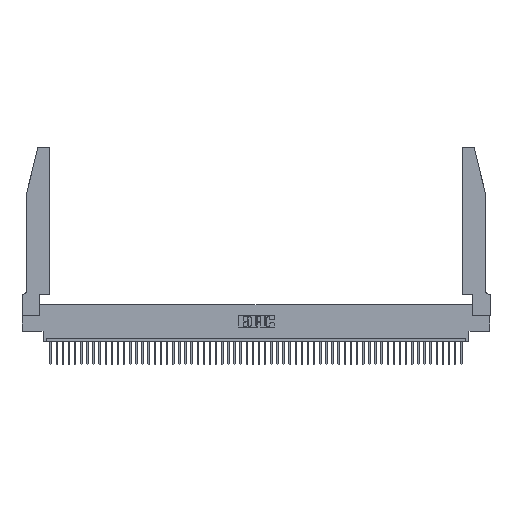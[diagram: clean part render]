
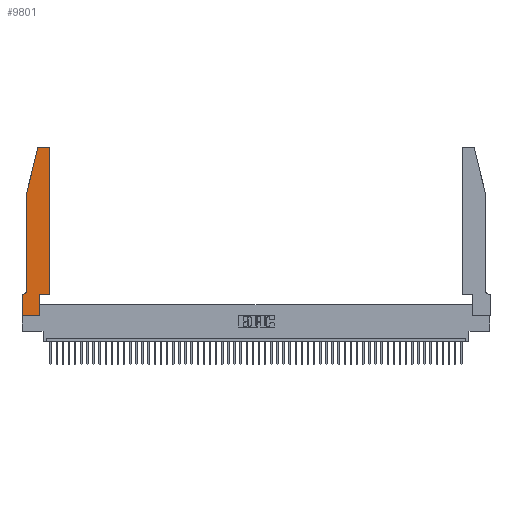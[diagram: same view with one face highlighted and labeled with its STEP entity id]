
A CAD part, top view. The second image highlights one B-rep face of the part: STEP entity #9801.
In plain terms, the highlighted planar face has unit normal (0, 0, 1).
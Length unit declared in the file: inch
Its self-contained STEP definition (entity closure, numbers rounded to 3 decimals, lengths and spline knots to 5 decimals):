
#990 = CARTESIAN_POINT ( 'NONE',  ( 0.2605, 2.75, 0.37 ) ) ;
#1008 = DIRECTION ( 'NONE',  ( 1., 0., 0. ) ) ;
#2313 = ORIENTED_EDGE ( 'NONE', *, *, #16803, .T. ) ;
#2645 = CARTESIAN_POINT ( 'NONE',  ( 0.0755, 0.42, 0.37 ) ) ;
#2916 = VECTOR ( 'NONE', #13796, 39.37008 ) ;
#2956 = DIRECTION ( 'NONE',  ( 0., 1., 0. ) ) ;
#4282 = VECTOR ( 'NONE', #18488, 39.37008 ) ;
#5084 = EDGE_CURVE ( 'NONE', #20012, #34031, #16557, .T. ) ;
#5178 = EDGE_CURVE ( 'NONE', #34031, #5713, #45083, .T. ) ;
#5594 = DIRECTION ( 'NONE',  ( 0., 0., 1. ) ) ;
#5713 = VERTEX_POINT ( 'NONE', #12394 ) ;
#6155 = EDGE_CURVE ( 'NONE', #8151, #35009, #12959, .T. ) ;
#7456 = VECTOR ( 'NONE', #34165, 39.37008 ) ;
#8151 = VERTEX_POINT ( 'NONE', #10518 ) ;
#9075 = CARTESIAN_POINT ( 'NONE',  ( 0.2865, 0.35, 0.37 ) ) ;
#9334 = CARTESIAN_POINT ( 'NONE',  ( 0., 0., 0.37 ) ) ;
#9801 = ADVANCED_FACE ( 'NONE', ( #12175 ), #47175, .T. ) ;
#10412 = ORIENTED_EDGE ( 'NONE', *, *, #41816, .T. ) ;
#10518 = CARTESIAN_POINT ( 'NONE',  ( 0.0755, 2., 0.37 ) ) ;
#11980 = CARTESIAN_POINT ( 'NONE',  ( 0.4205, 2.75, 0.37 ) ) ;
#12064 = CIRCLE ( 'NONE', #22218, 0.03 ) ;
#12175 = FACE_OUTER_BOUND ( 'NONE', #51676, .T. ) ;
#12394 = CARTESIAN_POINT ( 'NONE',  ( 0., 0., 0.37 ) ) ;
#12959 = LINE ( 'NONE', #13630, #49100 ) ;
#13179 = EDGE_CURVE ( 'NONE', #5713, #50501, #47459, .T. ) ;
#13371 = EDGE_CURVE ( 'NONE', #25497, #16295, #32127, .T. ) ;
#13630 = CARTESIAN_POINT ( 'NONE',  ( 0.0755, 2., 0.37 ) ) ;
#13796 = DIRECTION ( 'NONE',  ( 1., 0., 0. ) ) ;
#14965 = LINE ( 'NONE', #47362, #35889 ) ;
#16295 = VERTEX_POINT ( 'NONE', #37887 ) ;
#16557 = LINE ( 'NONE', #52510, #31771 ) ;
#16803 = EDGE_CURVE ( 'NONE', #27296, #44970, #12064, .T. ) ;
#17309 = VECTOR ( 'NONE', #37093, 39.37008 ) ;
#17641 = CARTESIAN_POINT ( 'NONE',  ( 0.4205, 2.72, 0.37 ) ) ;
#18488 = DIRECTION ( 'NONE',  ( -0.239, -0.971, 0. ) ) ;
#18759 = CARTESIAN_POINT ( 'NONE',  ( 0.2865, 0., 0.37 ) ) ;
#19141 = CARTESIAN_POINT ( 'NONE',  ( 0., 0.35, 0.37 ) ) ;
#20012 = VERTEX_POINT ( 'NONE', #29190 ) ;
#20167 = DIRECTION ( 'NONE',  ( -1., 0., 0. ) ) ;
#20711 = LINE ( 'NONE', #990, #7456 ) ;
#21055 = CIRCLE ( 'NONE', #21186, 0.03 ) ;
#21186 = AXIS2_PLACEMENT_3D ( 'NONE', #29906, #5594, #1008 ) ;
#21304 = ORIENTED_EDGE ( 'NONE', *, *, #41875, .T. ) ;
#21490 = DIRECTION ( 'NONE',  ( 1., 0., 0. ) ) ;
#22218 = AXIS2_PLACEMENT_3D ( 'NONE', #17641, #25330, #21490 ) ;
#22264 = CARTESIAN_POINT ( 'NONE',  ( 0.4505, 0.35, 0.37 ) ) ;
#22865 = VECTOR ( 'NONE', #39951, 39.37008 ) ;
#23477 = EDGE_CURVE ( 'NONE', #44970, #25461, #20711, .T. ) ;
#25154 = ORIENTED_EDGE ( 'NONE', *, *, #5178, .T. ) ;
#25330 = DIRECTION ( 'NONE',  ( 0., 0., 1. ) ) ;
#25461 = VERTEX_POINT ( 'NONE', #40736 ) ;
#25497 = VERTEX_POINT ( 'NONE', #9075 ) ;
#26162 = CARTESIAN_POINT ( 'NONE',  ( 0.0755, 2., 0.37 ) ) ;
#26347 = EDGE_CURVE ( 'NONE', #50501, #25497, #38945, .T. ) ;
#26525 = ORIENTED_EDGE ( 'NONE', *, *, #23477, .T. ) ;
#26849 = DIRECTION ( 'NONE',  ( 1., 0., 0. ) ) ;
#27296 = VERTEX_POINT ( 'NONE', #30153 ) ;
#28089 = DIRECTION ( 'NONE',  ( 0., 0., -1. ) ) ;
#28155 = AXIS2_PLACEMENT_3D ( 'NONE', #34890, #42731, #26849 ) ;
#28504 = EDGE_CURVE ( 'NONE', #42590, #8151, #43123, .T. ) ;
#28607 = ORIENTED_EDGE ( 'NONE', *, *, #13179, .T. ) ;
#29190 = CARTESIAN_POINT ( 'NONE',  ( 0.0055, 0.35, 0.37 ) ) ;
#29906 = CARTESIAN_POINT ( 'NONE',  ( 0.284, 2.72, 0.37 ) ) ;
#30118 = AXIS2_PLACEMENT_3D ( 'NONE', #52169, #28089, #20167 ) ;
#30146 = ORIENTED_EDGE ( 'NONE', *, *, #6155, .T. ) ;
#30153 = CARTESIAN_POINT ( 'NONE',  ( 0.4505, 2.72, 0.37 ) ) ;
#30626 = DIRECTION ( 'NONE',  ( 0., -1., 0. ) ) ;
#31771 = VECTOR ( 'NONE', #42269, 39.37008 ) ;
#32127 = LINE ( 'NONE', #22264, #2916 ) ;
#34031 = VERTEX_POINT ( 'NONE', #19141 ) ;
#34165 = DIRECTION ( 'NONE',  ( -1., 0., 0. ) ) ;
#34890 = CARTESIAN_POINT ( 'NONE',  ( 0., 0.35, 0.37 ) ) ;
#35009 = VERTEX_POINT ( 'NONE', #2645 ) ;
#35889 = VECTOR ( 'NONE', #2956, 39.37008 ) ;
#37093 = DIRECTION ( 'NONE',  ( 0., 1., 0. ) ) ;
#37213 = ORIENTED_EDGE ( 'NONE', *, *, #26347, .T. ) ;
#37818 = ORIENTED_EDGE ( 'NONE', *, *, #13371, .T. ) ;
#37887 = CARTESIAN_POINT ( 'NONE',  ( 0.4505, 0.35, 0.37 ) ) ;
#38945 = LINE ( 'NONE', #45955, #17309 ) ;
#39951 = DIRECTION ( 'NONE',  ( 0., -1., 0. ) ) ;
#40321 = CARTESIAN_POINT ( 'NONE',  ( 0., 0., 0.37 ) ) ;
#40736 = CARTESIAN_POINT ( 'NONE',  ( 0.284, 2.75, 0.37 ) ) ;
#40923 = CARTESIAN_POINT ( 'NONE',  ( 0.25487, 2.72718, 0.37 ) ) ;
#41816 = EDGE_CURVE ( 'NONE', #16295, #27296, #14965, .T. ) ;
#41875 = EDGE_CURVE ( 'NONE', #35009, #20012, #45363, .T. ) ;
#42269 = DIRECTION ( 'NONE',  ( -1., 0., 0. ) ) ;
#42590 = VERTEX_POINT ( 'NONE', #40923 ) ;
#42731 = DIRECTION ( 'NONE',  ( 0., 0., 1. ) ) ;
#43123 = LINE ( 'NONE', #26162, #4282 ) ;
#43734 = ORIENTED_EDGE ( 'NONE', *, *, #49555, .T. ) ;
#44881 = VECTOR ( 'NONE', #50532, 39.37008 ) ;
#44970 = VERTEX_POINT ( 'NONE', #11980 ) ;
#45083 = LINE ( 'NONE', #40321, #22865 ) ;
#45363 = CIRCLE ( 'NONE', #30118, 0.07 ) ;
#45955 = CARTESIAN_POINT ( 'NONE',  ( 0.2865, 0.35, 0.37 ) ) ;
#46039 = ORIENTED_EDGE ( 'NONE', *, *, #5084, .T. ) ;
#47175 = PLANE ( 'NONE',  #28155 ) ;
#47362 = CARTESIAN_POINT ( 'NONE',  ( 0.4505, 0.35, 0.37 ) ) ;
#47459 = LINE ( 'NONE', #9334, #44881 ) ;
#48641 = ORIENTED_EDGE ( 'NONE', *, *, #28504, .T. ) ;
#49100 = VECTOR ( 'NONE', #30626, 39.37008 ) ;
#49555 = EDGE_CURVE ( 'NONE', #25461, #42590, #21055, .T. ) ;
#50501 = VERTEX_POINT ( 'NONE', #18759 ) ;
#50532 = DIRECTION ( 'NONE',  ( 1., 0., 0. ) ) ;
#51676 = EDGE_LOOP ( 'NONE', ( #26525, #43734, #48641, #30146, #21304, #46039, #25154, #28607, #37213, #37818, #10412, #2313 ) ) ;
#52169 = CARTESIAN_POINT ( 'NONE',  ( 0.0055, 0.42, 0.37 ) ) ;
#52510 = CARTESIAN_POINT ( 'NONE',  ( 0.0755, 0.35, 0.37 ) ) ;
